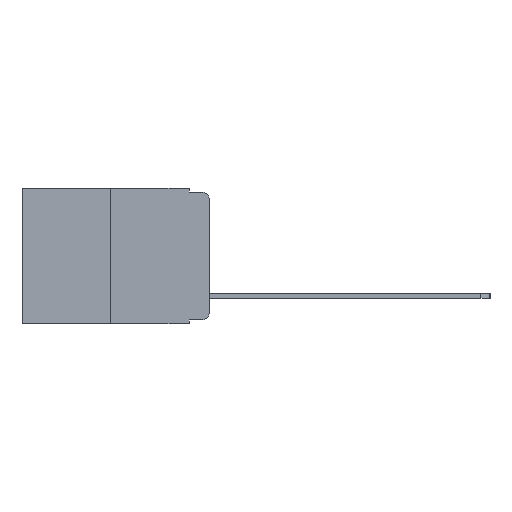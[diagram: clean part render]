
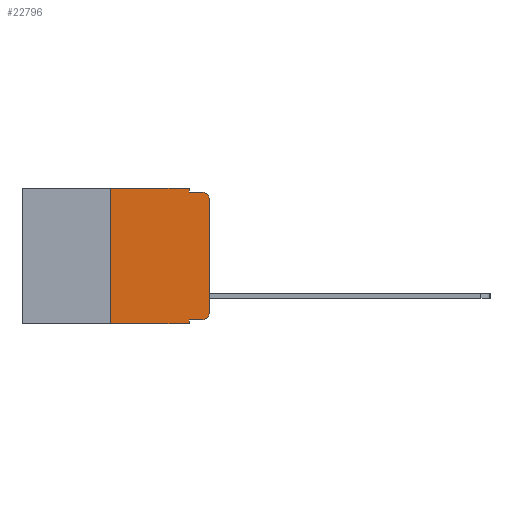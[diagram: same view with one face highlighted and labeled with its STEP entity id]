
A CAD part, left-side view. The second image highlights one B-rep face of the part: STEP entity #22796.
In plain terms, the highlighted planar face has unit normal (-1, 0, 0).
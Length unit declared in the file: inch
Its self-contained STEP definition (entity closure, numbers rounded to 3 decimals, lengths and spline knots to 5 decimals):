
#1011 = VERTEX_POINT ( 'NONE', #21879 ) ;
#1079 = EDGE_CURVE ( 'NONE', #19344, #6812, #7421, .T. ) ;
#1618 = LINE ( 'NONE', #10999, #15678 ) ;
#2348 = EDGE_CURVE ( 'NONE', #19879, #19344, #11072, .T. ) ;
#2397 = CIRCLE ( 'NONE', #12573, 0.02 ) ;
#2835 = VECTOR ( 'NONE', #21464, 39.37008 ) ;
#2889 = VECTOR ( 'NONE', #19305, 39.37008 ) ;
#3059 = LINE ( 'NONE', #4647, #21319 ) ;
#3338 = CARTESIAN_POINT ( 'NONE',  ( 0., 0.473, 0. ) ) ;
#4309 = CARTESIAN_POINT ( 'NONE',  ( 0., 0.051, -0.333 ) ) ;
#4502 = CARTESIAN_POINT ( 'NONE',  ( 0., 0., 0. ) ) ;
#4647 = CARTESIAN_POINT ( 'NONE',  ( 0., 0.473, 0. ) ) ;
#5259 = ORIENTED_EDGE ( 'NONE', *, *, #11427, .T. ) ;
#5485 = CARTESIAN_POINT ( 'NONE',  ( 0., 0.051, 0. ) ) ;
#5548 = DIRECTION ( 'NONE',  ( 0., 0., -1. ) ) ;
#5634 = ORIENTED_EDGE ( 'NONE', *, *, #12628, .T. ) ;
#5861 = FACE_OUTER_BOUND ( 'NONE', #12910, .T. ) ;
#5968 = ORIENTED_EDGE ( 'NONE', *, *, #17484, .F. ) ;
#6004 = VECTOR ( 'NONE', #13780, 39.37008 ) ;
#6080 = ORIENTED_EDGE ( 'NONE', *, *, #6378, .T. ) ;
#6206 = VECTOR ( 'NONE', #6363, 39.37008 ) ;
#6363 = DIRECTION ( 'NONE',  ( 0., 0., 1. ) ) ;
#6378 = EDGE_CURVE ( 'NONE', #16869, #9129, #7182, .T. ) ;
#6441 = ORIENTED_EDGE ( 'NONE', *, *, #18704, .F. ) ;
#6512 = DIRECTION ( 'NONE',  ( 0., -1., 0. ) ) ;
#6640 = DIRECTION ( 'NONE',  ( -1., 0., 0. ) ) ;
#6655 = ORIENTED_EDGE ( 'NONE', *, *, #7479, .F. ) ;
#6679 = ORIENTED_EDGE ( 'NONE', *, *, #19916, .F. ) ;
#6812 = VERTEX_POINT ( 'NONE', #11817 ) ;
#6956 = CARTESIAN_POINT ( 'NONE',  ( 0., 0.473, -0.343 ) ) ;
#7082 = DIRECTION ( 'NONE',  ( 0., 0., -1. ) ) ;
#7182 = LINE ( 'NONE', #6956, #2835 ) ;
#7226 = ORIENTED_EDGE ( 'NONE', *, *, #23522, .F. ) ;
#7421 = CIRCLE ( 'NONE', #12766, 0.02 ) ;
#7479 = EDGE_CURVE ( 'NONE', #20054, #22962, #3059, .T. ) ;
#8056 = ORIENTED_EDGE ( 'NONE', *, *, #1079, .T. ) ;
#8073 = CARTESIAN_POINT ( 'NONE',  ( 0., 0.051, -0.343 ) ) ;
#8288 = CARTESIAN_POINT ( 'NONE',  ( 0., 0.25, 0. ) ) ;
#8434 = CARTESIAN_POINT ( 'NONE',  ( 0., 0.051, -0.333 ) ) ;
#8516 = LINE ( 'NONE', #23606, #11656 ) ;
#9129 = VERTEX_POINT ( 'NONE', #8073 ) ;
#9214 = ORIENTED_EDGE ( 'NONE', *, *, #2348, .T. ) ;
#10999 = CARTESIAN_POINT ( 'NONE',  ( 0., 0.051, 0. ) ) ;
#11012 = DIRECTION ( 'NONE',  ( 0., 0., -1. ) ) ;
#11072 = LINE ( 'NONE', #4502, #6206 ) ;
#11389 = CARTESIAN_POINT ( 'NONE',  ( 0., 0.25, 0. ) ) ;
#11427 = EDGE_CURVE ( 'NONE', #1011, #19879, #2397, .T. ) ;
#11656 = VECTOR ( 'NONE', #12872, 39.37008 ) ;
#11817 = CARTESIAN_POINT ( 'NONE',  ( 0., 0.02, -0.01 ) ) ;
#12016 = LINE ( 'NONE', #8288, #6004 ) ;
#12573 = AXIS2_PLACEMENT_3D ( 'NONE', #17526, #6640, #19366 ) ;
#12628 = EDGE_CURVE ( 'NONE', #22160, #1011, #13241, .T. ) ;
#12766 = AXIS2_PLACEMENT_3D ( 'NONE', #22299, #21627, #21025 ) ;
#12872 = DIRECTION ( 'NONE',  ( 0., -1., 0. ) ) ;
#12910 = EDGE_LOOP ( 'NONE', ( #9214, #8056, #7226, #6679, #6655, #6441, #6080, #5968, #5634, #5259 ) ) ;
#13241 = LINE ( 'NONE', #8434, #2889 ) ;
#13780 = DIRECTION ( 'NONE',  ( 0., 0., 1. ) ) ;
#14285 = AXIS2_PLACEMENT_3D ( 'NONE', #3338, #17968, #7082 ) ;
#14336 = PLANE ( 'NONE',  #14285 ) ;
#14538 = CARTESIAN_POINT ( 'NONE',  ( 0., 0.25, -0.343 ) ) ;
#15678 = VECTOR ( 'NONE', #5548, 39.37008 ) ;
#16322 = CARTESIAN_POINT ( 'NONE',  ( 0., 0., -0.313 ) ) ;
#16869 = VERTEX_POINT ( 'NONE', #14538 ) ;
#17457 = CARTESIAN_POINT ( 'NONE',  ( 0., 0., -0.03 ) ) ;
#17484 = EDGE_CURVE ( 'NONE', #22160, #9129, #19987, .T. ) ;
#17526 = CARTESIAN_POINT ( 'NONE',  ( 0., 0.02, -0.313 ) ) ;
#17968 = DIRECTION ( 'NONE',  ( 1., 0., 0. ) ) ;
#18704 = EDGE_CURVE ( 'NONE', #16869, #20054, #12016, .T. ) ;
#19305 = DIRECTION ( 'NONE',  ( 0., -1., 0. ) ) ;
#19344 = VERTEX_POINT ( 'NONE', #17457 ) ;
#19366 = DIRECTION ( 'NONE',  ( 0., 0., -1. ) ) ;
#19879 = VERTEX_POINT ( 'NONE', #16322 ) ;
#19916 = EDGE_CURVE ( 'NONE', #22962, #20579, #1618, .T. ) ;
#19987 = LINE ( 'NONE', #5485, #23643 ) ;
#20054 = VERTEX_POINT ( 'NONE', #11389 ) ;
#20579 = VERTEX_POINT ( 'NONE', #22036 ) ;
#21025 = DIRECTION ( 'NONE',  ( 0., 0., -1. ) ) ;
#21319 = VECTOR ( 'NONE', #6512, 39.37008 ) ;
#21464 = DIRECTION ( 'NONE',  ( 0., -1., 0. ) ) ;
#21627 = DIRECTION ( 'NONE',  ( -1., 0., 0. ) ) ;
#21879 = CARTESIAN_POINT ( 'NONE',  ( 0., 0.02, -0.333 ) ) ;
#22036 = CARTESIAN_POINT ( 'NONE',  ( 0., 0.051, -0.01 ) ) ;
#22062 = CARTESIAN_POINT ( 'NONE',  ( 0., 0.051, 0. ) ) ;
#22160 = VERTEX_POINT ( 'NONE', #4309 ) ;
#22299 = CARTESIAN_POINT ( 'NONE',  ( 0., 0.02, -0.03 ) ) ;
#22796 = ADVANCED_FACE ( 'NONE', ( #5861 ), #14336, .F. ) ;
#22962 = VERTEX_POINT ( 'NONE', #22062 ) ;
#23522 = EDGE_CURVE ( 'NONE', #20579, #6812, #8516, .T. ) ;
#23606 = CARTESIAN_POINT ( 'NONE',  ( 0., 0.051, -0.01 ) ) ;
#23643 = VECTOR ( 'NONE', #11012, 39.37008 ) ;
